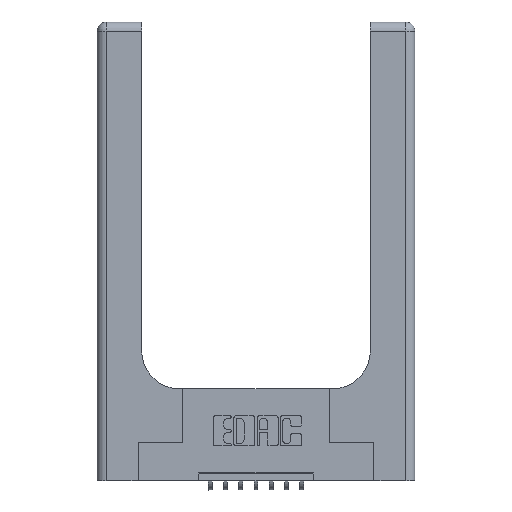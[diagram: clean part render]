
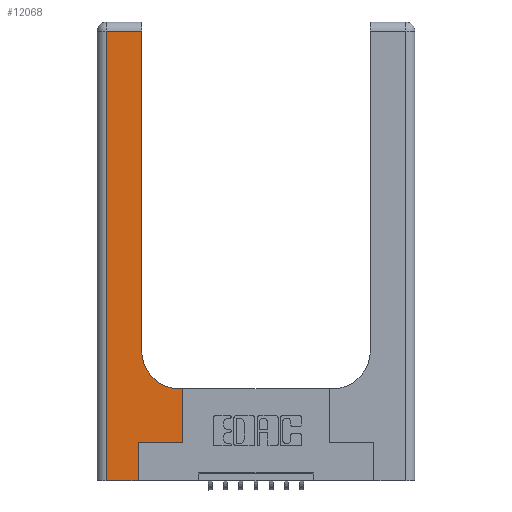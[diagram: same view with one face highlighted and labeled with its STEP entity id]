
A CAD part, top view. The second image highlights one B-rep face of the part: STEP entity #12068.
In plain terms, the highlighted planar face has unit normal (0, 0, 1).
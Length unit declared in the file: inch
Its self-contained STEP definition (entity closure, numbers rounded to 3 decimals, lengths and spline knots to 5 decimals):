
#236 = LINE ( 'NONE', #13948, #1711 ) ;
#514 = ORIENTED_EDGE ( 'NONE', *, *, #5478, .T. ) ;
#521 = CARTESIAN_POINT ( 'NONE',  ( 0.269, 0., 0.37 ) ) ;
#702 = CARTESIAN_POINT ( 'NONE',  ( 0.269, 0., 0.37 ) ) ;
#908 = DIRECTION ( 'NONE',  ( -1., 0., 0. ) ) ;
#985 = LINE ( 'NONE', #10170, #13167 ) ;
#1036 = CARTESIAN_POINT ( 'NONE',  ( 0.2915, 3., 0.37 ) ) ;
#1263 = EDGE_CURVE ( 'NONE', #14644, #1524, #6982, .T. ) ;
#1524 = VERTEX_POINT ( 'NONE', #9390 ) ;
#1593 = EDGE_CURVE ( 'NONE', #15061, #6796, #12509, .T. ) ;
#1646 = LINE ( 'NONE', #6544, #13823 ) ;
#1711 = VECTOR ( 'NONE', #2257, 39.37008 ) ;
#1974 = DIRECTION ( 'NONE',  ( 1., 0., 0. ) ) ;
#2144 = VECTOR ( 'NONE', #908, 39.37008 ) ;
#2237 = ORIENTED_EDGE ( 'NONE', *, *, #12524, .T. ) ;
#2257 = DIRECTION ( 'NONE',  ( 0., -1., 0. ) ) ;
#2276 = DIRECTION ( 'NONE',  ( 1., 0., 0. ) ) ;
#2371 = AXIS2_PLACEMENT_3D ( 'NONE', #8033, #15128, #12792 ) ;
#3140 = CARTESIAN_POINT ( 'NONE',  ( 0.2915, 0.6, 0.37 ) ) ;
#3292 = LINE ( 'NONE', #9822, #11939 ) ;
#3468 = EDGE_CURVE ( 'NONE', #6796, #14644, #6738, .T. ) ;
#3795 = VERTEX_POINT ( 'NONE', #4528 ) ;
#4528 = CARTESIAN_POINT ( 'NONE',  ( 0.269, 0.25, 0.37 ) ) ;
#4604 = ORIENTED_EDGE ( 'NONE', *, *, #8301, .T. ) ;
#4736 = LINE ( 'NONE', #1036, #8784 ) ;
#5478 = EDGE_CURVE ( 'NONE', #1524, #12177, #4736, .T. ) ;
#5855 = CARTESIAN_POINT ( 'NONE',  ( 0.5415, 0.85, 0.37 ) ) ;
#6245 = VECTOR ( 'NONE', #11071, 39.37008 ) ;
#6385 = DIRECTION ( 'NONE',  ( 0., 1., 0. ) ) ;
#6541 = VECTOR ( 'NONE', #6385, 39.37008 ) ;
#6544 = CARTESIAN_POINT ( 'NONE',  ( 0.269, 0.25, 0.37 ) ) ;
#6738 = LINE ( 'NONE', #3140, #2144 ) ;
#6796 = VERTEX_POINT ( 'NONE', #12265 ) ;
#6858 = PLANE ( 'NONE',  #2371 ) ;
#6980 = EDGE_CURVE ( 'NONE', #9087, #3795, #9691, .T. ) ;
#6982 = CIRCLE ( 'NONE', #12542, 0.25 ) ;
#6987 = DIRECTION ( 'NONE',  ( 0., 0., -1. ) ) ;
#6993 = ORIENTED_EDGE ( 'NONE', *, *, #1593, .T. ) ;
#7200 = CARTESIAN_POINT ( 'NONE',  ( 0.5415, 0.6, 0.37 ) ) ;
#7236 = ORIENTED_EDGE ( 'NONE', *, *, #1263, .T. ) ;
#7330 = ORIENTED_EDGE ( 'NONE', *, *, #3468, .T. ) ;
#8033 = CARTESIAN_POINT ( 'NONE',  ( 0., 3., 0.37 ) ) ;
#8195 = EDGE_CURVE ( 'NONE', #8835, #9087, #985, .T. ) ;
#8301 = EDGE_CURVE ( 'NONE', #8566, #8835, #236, .T. ) ;
#8382 = CARTESIAN_POINT ( 'NONE',  ( 0.5585, 0.25, 0.37 ) ) ;
#8472 = ORIENTED_EDGE ( 'NONE', *, *, #8195, .T. ) ;
#8566 = VERTEX_POINT ( 'NONE', #13344 ) ;
#8784 = VECTOR ( 'NONE', #9232, 39.37008 ) ;
#8835 = VERTEX_POINT ( 'NONE', #13781 ) ;
#9087 = VERTEX_POINT ( 'NONE', #702 ) ;
#9232 = DIRECTION ( 'NONE',  ( 0., 1., 0. ) ) ;
#9390 = CARTESIAN_POINT ( 'NONE',  ( 0.2915, 0.85, 0.37 ) ) ;
#9691 = LINE ( 'NONE', #521, #6541 ) ;
#9822 = CARTESIAN_POINT ( 'NONE',  ( 0., 2.94, 0.37 ) ) ;
#9904 = CARTESIAN_POINT ( 'NONE',  ( 0.5585, 0.25, 0.37 ) ) ;
#10170 = CARTESIAN_POINT ( 'NONE',  ( 0., 0., 0.37 ) ) ;
#10564 = ORIENTED_EDGE ( 'NONE', *, *, #6980, .T. ) ;
#10813 = EDGE_CURVE ( 'NONE', #3795, #15061, #1646, .T. ) ;
#11071 = DIRECTION ( 'NONE',  ( 0., 1., 0. ) ) ;
#11551 = CARTESIAN_POINT ( 'NONE',  ( 0.2915, 2.94, 0.37 ) ) ;
#11848 = ORIENTED_EDGE ( 'NONE', *, *, #10813, .T. ) ;
#11939 = VECTOR ( 'NONE', #14749, 39.37008 ) ;
#11958 = FACE_OUTER_BOUND ( 'NONE', #14819, .T. ) ;
#12068 = ADVANCED_FACE ( 'NONE', ( #11958 ), #6858, .F. ) ;
#12177 = VERTEX_POINT ( 'NONE', #11551 ) ;
#12265 = CARTESIAN_POINT ( 'NONE',  ( 0.5585, 0.6, 0.37 ) ) ;
#12509 = LINE ( 'NONE', #9904, #6245 ) ;
#12524 = EDGE_CURVE ( 'NONE', #12177, #8566, #3292, .T. ) ;
#12542 = AXIS2_PLACEMENT_3D ( 'NONE', #5855, #6987, #2276 ) ;
#12792 = DIRECTION ( 'NONE',  ( -1., 0., 0. ) ) ;
#13167 = VECTOR ( 'NONE', #1974, 39.37008 ) ;
#13344 = CARTESIAN_POINT ( 'NONE',  ( 0.06, 2.94, 0.37 ) ) ;
#13781 = CARTESIAN_POINT ( 'NONE',  ( 0.06, 0., 0.37 ) ) ;
#13823 = VECTOR ( 'NONE', #14842, 39.37008 ) ;
#13948 = CARTESIAN_POINT ( 'NONE',  ( 0.06, 3., 0.37 ) ) ;
#14644 = VERTEX_POINT ( 'NONE', #7200 ) ;
#14749 = DIRECTION ( 'NONE',  ( -1., 0., 0. ) ) ;
#14819 = EDGE_LOOP ( 'NONE', ( #514, #2237, #4604, #8472, #10564, #11848, #6993, #7330, #7236 ) ) ;
#14842 = DIRECTION ( 'NONE',  ( 1., 0., 0. ) ) ;
#15061 = VERTEX_POINT ( 'NONE', #8382 ) ;
#15128 = DIRECTION ( 'NONE',  ( 0., 0., -1. ) ) ;
